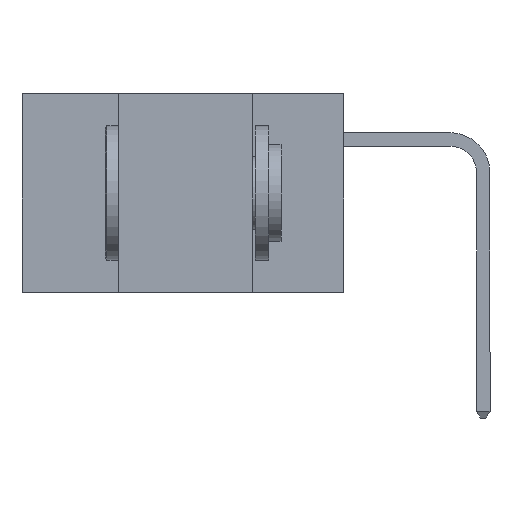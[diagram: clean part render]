
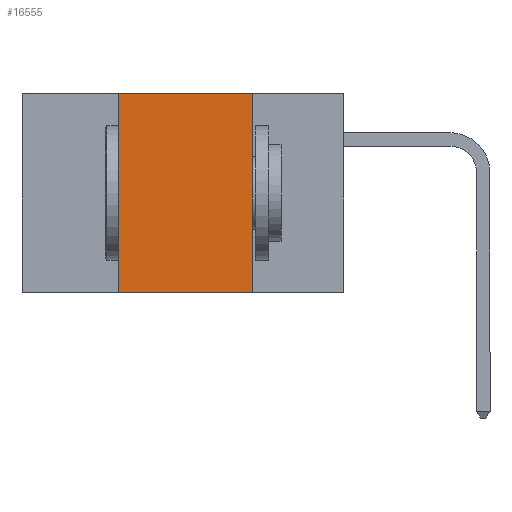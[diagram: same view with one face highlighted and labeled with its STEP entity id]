
A CAD part, left-side view. The second image highlights one B-rep face of the part: STEP entity #16555.
In plain terms, the highlighted planar face has unit normal (-1, 0, 0).
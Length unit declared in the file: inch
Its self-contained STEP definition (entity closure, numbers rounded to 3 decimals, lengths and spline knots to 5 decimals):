
#411 = DIRECTION ( 'NONE',  ( 0., 0., 1. ) ) ;
#526 = ORIENTED_EDGE ( 'NONE', *, *, #5736, .F. ) ;
#1076 = DIRECTION ( 'NONE',  ( 0., 0., -1. ) ) ;
#2176 = PLANE ( 'NONE',  #5404 ) ;
#2357 = VERTEX_POINT ( 'NONE', #9183 ) ;
#2682 = DIRECTION ( 'NONE',  ( 0., -1., 0. ) ) ;
#3956 = ORIENTED_EDGE ( 'NONE', *, *, #7859, .T. ) ;
#5048 = VECTOR ( 'NONE', #16157, 39.37008 ) ;
#5404 = AXIS2_PLACEMENT_3D ( 'NONE', #13259, #14833, #5538 ) ;
#5412 = VECTOR ( 'NONE', #1076, 39.37008 ) ;
#5538 = DIRECTION ( 'NONE',  ( 0., 0., -1. ) ) ;
#5736 = EDGE_CURVE ( 'NONE', #13629, #15617, #17336, .T. ) ;
#7859 = EDGE_CURVE ( 'NONE', #2357, #15617, #13326, .T. ) ;
#8196 = CARTESIAN_POINT ( 'NONE',  ( 0., 0.17, -0.37 ) ) ;
#8247 = ORIENTED_EDGE ( 'NONE', *, *, #10688, .F. ) ;
#9183 = CARTESIAN_POINT ( 'NONE',  ( 0., 0.42, -0.37 ) ) ;
#9690 = CARTESIAN_POINT ( 'NONE',  ( 0., 0.17, 0. ) ) ;
#9920 = EDGE_CURVE ( 'NONE', #2357, #18528, #11830, .T. ) ;
#10146 = CARTESIAN_POINT ( 'NONE',  ( 0., 0.42, 0. ) ) ;
#10654 = CARTESIAN_POINT ( 'NONE',  ( 0., 0.6, 0. ) ) ;
#10688 = EDGE_CURVE ( 'NONE', #18528, #13629, #18374, .T. ) ;
#11373 = ORIENTED_EDGE ( 'NONE', *, *, #9920, .F. ) ;
#11830 = LINE ( 'NONE', #10146, #20014 ) ;
#11937 = CARTESIAN_POINT ( 'NONE',  ( 0., 0.42, 0. ) ) ;
#13091 = CARTESIAN_POINT ( 'NONE',  ( 0., 0.6, -0.37 ) ) ;
#13259 = CARTESIAN_POINT ( 'NONE',  ( 0., 0.6, 0. ) ) ;
#13326 = LINE ( 'NONE', #13091, #5048 ) ;
#13629 = VERTEX_POINT ( 'NONE', #9690 ) ;
#14204 = VECTOR ( 'NONE', #2682, 39.37008 ) ;
#14833 = DIRECTION ( 'NONE',  ( 1., 0., 0. ) ) ;
#15617 = VERTEX_POINT ( 'NONE', #8196 ) ;
#16157 = DIRECTION ( 'NONE',  ( 0., -1., 0. ) ) ;
#16180 = EDGE_LOOP ( 'NONE', ( #526, #8247, #11373, #3956 ) ) ;
#16555 = ADVANCED_FACE ( 'NONE', ( #18636 ), #2176, .F. ) ;
#17336 = LINE ( 'NONE', #17890, #5412 ) ;
#17890 = CARTESIAN_POINT ( 'NONE',  ( 0., 0.17, 0. ) ) ;
#18374 = LINE ( 'NONE', #10654, #14204 ) ;
#18528 = VERTEX_POINT ( 'NONE', #11937 ) ;
#18636 = FACE_OUTER_BOUND ( 'NONE', #16180, .T. ) ;
#20014 = VECTOR ( 'NONE', #411, 39.37008 ) ;
